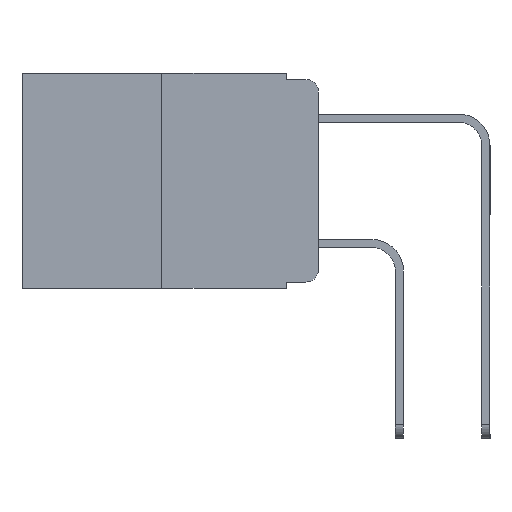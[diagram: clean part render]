
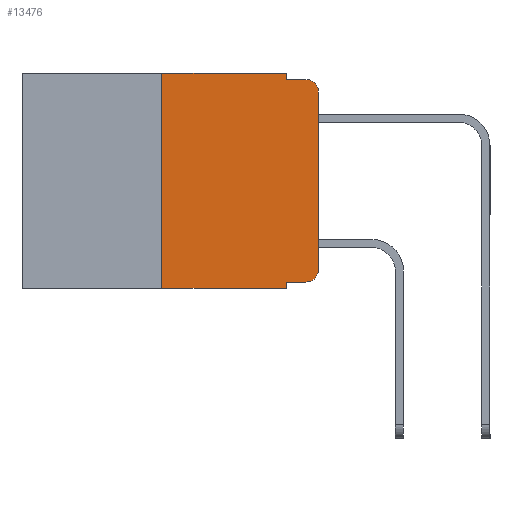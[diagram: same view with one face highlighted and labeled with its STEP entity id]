
A CAD part, left-side view. The second image highlights one B-rep face of the part: STEP entity #13476.
In plain terms, the highlighted planar face has unit normal (-1, 0, 0).
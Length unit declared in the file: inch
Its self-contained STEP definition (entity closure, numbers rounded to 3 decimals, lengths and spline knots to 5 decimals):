
#100 = DIRECTION ( 'NONE',  ( 0., 0., -1. ) ) ;
#321 = DIRECTION ( 'NONE',  ( 0., 0., 1. ) ) ;
#653 = EDGE_CURVE ( 'NONE', #916, #9569, #6867, .T. ) ;
#916 = VERTEX_POINT ( 'NONE', #17604 ) ;
#1687 = LINE ( 'NONE', #5295, #16713 ) ;
#1792 = CIRCLE ( 'NONE', #9440, 0.02 ) ;
#2255 = CARTESIAN_POINT ( 'NONE',  ( 0., 0., -0.313 ) ) ;
#2362 = ORIENTED_EDGE ( 'NONE', *, *, #18640, .F. ) ;
#2621 = DIRECTION ( 'NONE',  ( 1., 0., 0. ) ) ;
#2724 = EDGE_CURVE ( 'NONE', #9569, #9645, #14174, .T. ) ;
#3417 = ORIENTED_EDGE ( 'NONE', *, *, #653, .F. ) ;
#3818 = ORIENTED_EDGE ( 'NONE', *, *, #16692, .F. ) ;
#3895 = VERTEX_POINT ( 'NONE', #6247 ) ;
#3996 = ORIENTED_EDGE ( 'NONE', *, *, #5749, .T. ) ;
#4139 = DIRECTION ( 'NONE',  ( 0., -1., 0. ) ) ;
#4669 = VECTOR ( 'NONE', #6910, 39.37008 ) ;
#4730 = EDGE_CURVE ( 'NONE', #17379, #9645, #7966, .T. ) ;
#4892 = CARTESIAN_POINT ( 'NONE',  ( 0., 0.051, -0.333 ) ) ;
#5096 = CARTESIAN_POINT ( 'NONE',  ( 0., 0.051, 0. ) ) ;
#5157 = DIRECTION ( 'NONE',  ( 0., 0., -1. ) ) ;
#5277 = LINE ( 'NONE', #12842, #6182 ) ;
#5295 = CARTESIAN_POINT ( 'NONE',  ( 0., 0., 0. ) ) ;
#5405 = LINE ( 'NONE', #17874, #12626 ) ;
#5749 = EDGE_CURVE ( 'NONE', #18774, #17379, #1687, .T. ) ;
#6096 = VERTEX_POINT ( 'NONE', #16180 ) ;
#6182 = VECTOR ( 'NONE', #4139, 39.37008 ) ;
#6247 = CARTESIAN_POINT ( 'NONE',  ( 0., 0.02, -0.333 ) ) ;
#6380 = ORIENTED_EDGE ( 'NONE', *, *, #15744, .T. ) ;
#6399 = CARTESIAN_POINT ( 'NONE',  ( 0., 0.051, 0. ) ) ;
#6489 = ORIENTED_EDGE ( 'NONE', *, *, #18881, .T. ) ;
#6513 = DIRECTION ( 'NONE',  ( 0., -1., 0. ) ) ;
#6867 = LINE ( 'NONE', #6399, #7337 ) ;
#6910 = DIRECTION ( 'NONE',  ( 0., -1., 0. ) ) ;
#7025 = ORIENTED_EDGE ( 'NONE', *, *, #13831, .T. ) ;
#7190 = EDGE_LOOP ( 'NONE', ( #3996, #9067, #10058, #3417, #15933, #2362, #6489, #3818, #6380, #7025 ) ) ;
#7337 = VECTOR ( 'NONE', #13216, 39.37008 ) ;
#7966 = CIRCLE ( 'NONE', #10709, 0.02 ) ;
#8064 = CARTESIAN_POINT ( 'NONE',  ( 0., 0.02, -0.313 ) ) ;
#9009 = DIRECTION ( 'NONE',  ( -1., 0., 0. ) ) ;
#9067 = ORIENTED_EDGE ( 'NONE', *, *, #4730, .T. ) ;
#9222 = DIRECTION ( 'NONE',  ( 0., -1., 0. ) ) ;
#9440 = AXIS2_PLACEMENT_3D ( 'NONE', #8064, #18140, #9468 ) ;
#9468 = DIRECTION ( 'NONE',  ( 0., 0., -1. ) ) ;
#9569 = VERTEX_POINT ( 'NONE', #10533 ) ;
#9633 = CARTESIAN_POINT ( 'NONE',  ( 0., 0.25, 0. ) ) ;
#9641 = VERTEX_POINT ( 'NONE', #4892 ) ;
#9645 = VERTEX_POINT ( 'NONE', #16427 ) ;
#9819 = AXIS2_PLACEMENT_3D ( 'NONE', #11389, #2621, #12833 ) ;
#10058 = ORIENTED_EDGE ( 'NONE', *, *, #2724, .F. ) ;
#10533 = CARTESIAN_POINT ( 'NONE',  ( 0., 0.051, -0.01 ) ) ;
#10709 = AXIS2_PLACEMENT_3D ( 'NONE', #17688, #9009, #100 ) ;
#11389 = CARTESIAN_POINT ( 'NONE',  ( 0., 0.473, 0. ) ) ;
#11593 = LINE ( 'NONE', #5096, #15387 ) ;
#12276 = CARTESIAN_POINT ( 'NONE',  ( 0., 0.473, 0. ) ) ;
#12626 = VECTOR ( 'NONE', #321, 39.37008 ) ;
#12833 = DIRECTION ( 'NONE',  ( 0., 0., -1. ) ) ;
#12842 = CARTESIAN_POINT ( 'NONE',  ( 0., 0.051, -0.333 ) ) ;
#12944 = VECTOR ( 'NONE', #6513, 39.37008 ) ;
#13216 = DIRECTION ( 'NONE',  ( 0., 0., -1. ) ) ;
#13266 = EDGE_CURVE ( 'NONE', #17079, #916, #16287, .T. ) ;
#13476 = ADVANCED_FACE ( 'NONE', ( #15047 ), #17021, .F. ) ;
#13702 = VECTOR ( 'NONE', #9222, 39.37008 ) ;
#13831 = EDGE_CURVE ( 'NONE', #3895, #18774, #1792, .T. ) ;
#13952 = DIRECTION ( 'NONE',  ( 0., 0., 1. ) ) ;
#14174 = LINE ( 'NONE', #14904, #13702 ) ;
#14663 = CARTESIAN_POINT ( 'NONE',  ( 0., 0.051, -0.343 ) ) ;
#14904 = CARTESIAN_POINT ( 'NONE',  ( 0., 0.051, -0.01 ) ) ;
#15047 = FACE_OUTER_BOUND ( 'NONE', #7190, .T. ) ;
#15387 = VECTOR ( 'NONE', #5157, 39.37008 ) ;
#15744 = EDGE_CURVE ( 'NONE', #9641, #3895, #5277, .T. ) ;
#15933 = ORIENTED_EDGE ( 'NONE', *, *, #13266, .F. ) ;
#15968 = VERTEX_POINT ( 'NONE', #14663 ) ;
#16180 = CARTESIAN_POINT ( 'NONE',  ( 0., 0.25, -0.343 ) ) ;
#16287 = LINE ( 'NONE', #12276, #12944 ) ;
#16427 = CARTESIAN_POINT ( 'NONE',  ( 0., 0.02, -0.01 ) ) ;
#16692 = EDGE_CURVE ( 'NONE', #9641, #15968, #11593, .T. ) ;
#16713 = VECTOR ( 'NONE', #13952, 39.37008 ) ;
#16988 = CARTESIAN_POINT ( 'NONE',  ( 0., 0.473, -0.343 ) ) ;
#17021 = PLANE ( 'NONE',  #9819 ) ;
#17079 = VERTEX_POINT ( 'NONE', #9633 ) ;
#17379 = VERTEX_POINT ( 'NONE', #17550 ) ;
#17550 = CARTESIAN_POINT ( 'NONE',  ( 0., 0., -0.03 ) ) ;
#17604 = CARTESIAN_POINT ( 'NONE',  ( 0., 0.051, 0. ) ) ;
#17688 = CARTESIAN_POINT ( 'NONE',  ( 0., 0.02, -0.03 ) ) ;
#17874 = CARTESIAN_POINT ( 'NONE',  ( 0., 0.25, 0. ) ) ;
#17999 = LINE ( 'NONE', #16988, #4669 ) ;
#18140 = DIRECTION ( 'NONE',  ( -1., 0., 0. ) ) ;
#18640 = EDGE_CURVE ( 'NONE', #6096, #17079, #5405, .T. ) ;
#18774 = VERTEX_POINT ( 'NONE', #2255 ) ;
#18881 = EDGE_CURVE ( 'NONE', #6096, #15968, #17999, .T. ) ;
